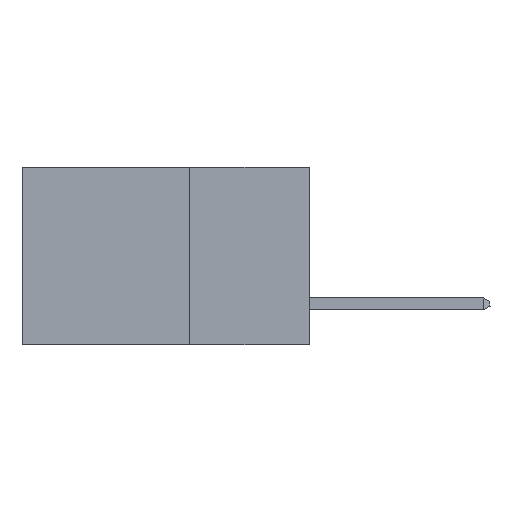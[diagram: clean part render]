
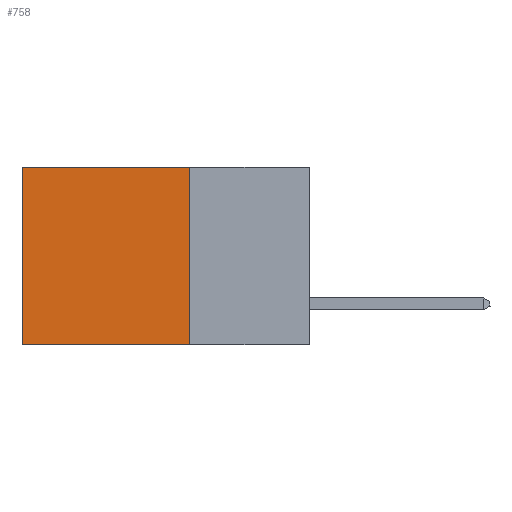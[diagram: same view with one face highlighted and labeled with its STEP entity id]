
A CAD part, left-side view. The second image highlights one B-rep face of the part: STEP entity #758.
In plain terms, the highlighted planar face has unit normal (-1, 0, 0).
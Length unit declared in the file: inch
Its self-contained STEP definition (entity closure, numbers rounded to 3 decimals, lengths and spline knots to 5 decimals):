
#326 = ORIENTED_EDGE ( 'NONE', *, *, #2407, .F. ) ;
#352 = VERTEX_POINT ( 'NONE', #2207 ) ;
#403 = CARTESIAN_POINT ( 'NONE',  ( 0.2875, 0.6, -0.37 ) ) ;
#758 = ADVANCED_FACE ( 'NONE', ( #17555 ), #6204, .F. ) ;
#1435 = VERTEX_POINT ( 'NONE', #6891 ) ;
#1757 = DIRECTION ( 'NONE',  ( 0., 0., -1. ) ) ;
#2174 = VECTOR ( 'NONE', #9789, 39.37008 ) ;
#2207 = CARTESIAN_POINT ( 'NONE',  ( 0.2875, 0.25, -0.37 ) ) ;
#2407 = EDGE_CURVE ( 'NONE', #352, #15777, #14944, .T. ) ;
#3303 = CARTESIAN_POINT ( 'NONE',  ( 0.2875, 0.25, 0. ) ) ;
#6085 = CARTESIAN_POINT ( 'NONE',  ( 0.2875, 0.25, 0. ) ) ;
#6204 = PLANE ( 'NONE',  #9492 ) ;
#6891 = CARTESIAN_POINT ( 'NONE',  ( 0.2875, 0.6, 0. ) ) ;
#6972 = LINE ( 'NONE', #3303, #2174 ) ;
#7022 = VECTOR ( 'NONE', #19555, 39.37008 ) ;
#7143 = DIRECTION ( 'NONE',  ( 0., 1., 0. ) ) ;
#7498 = EDGE_CURVE ( 'NONE', #1435, #15777, #16164, .T. ) ;
#8388 = CARTESIAN_POINT ( 'NONE',  ( 0.2875, 0.6, 0. ) ) ;
#9492 = AXIS2_PLACEMENT_3D ( 'NONE', #11681, #16072, #14426 ) ;
#9623 = CARTESIAN_POINT ( 'NONE',  ( 0.2875, 0.25, 0. ) ) ;
#9789 = DIRECTION ( 'NONE',  ( 0., 1., 0. ) ) ;
#10843 = EDGE_LOOP ( 'NONE', ( #18741, #326, #12575, #13223 ) ) ;
#11681 = CARTESIAN_POINT ( 'NONE',  ( 0.2875, 0.25, 0. ) ) ;
#12229 = VECTOR ( 'NONE', #1757, 39.37008 ) ;
#12575 = ORIENTED_EDGE ( 'NONE', *, *, #15576, .F. ) ;
#13223 = ORIENTED_EDGE ( 'NONE', *, *, #17467, .T. ) ;
#14426 = DIRECTION ( 'NONE',  ( 0., 0., -1. ) ) ;
#14427 = VERTEX_POINT ( 'NONE', #6085 ) ;
#14944 = LINE ( 'NONE', #16896, #15486 ) ;
#15486 = VECTOR ( 'NONE', #7143, 39.37008 ) ;
#15576 = EDGE_CURVE ( 'NONE', #14427, #352, #19356, .T. ) ;
#15777 = VERTEX_POINT ( 'NONE', #403 ) ;
#16072 = DIRECTION ( 'NONE',  ( 1., 0., 0. ) ) ;
#16164 = LINE ( 'NONE', #8388, #7022 ) ;
#16896 = CARTESIAN_POINT ( 'NONE',  ( 0.2875, 0.25, -0.37 ) ) ;
#17467 = EDGE_CURVE ( 'NONE', #14427, #1435, #6972, .T. ) ;
#17555 = FACE_OUTER_BOUND ( 'NONE', #10843, .T. ) ;
#18741 = ORIENTED_EDGE ( 'NONE', *, *, #7498, .T. ) ;
#19356 = LINE ( 'NONE', #9623, #12229 ) ;
#19555 = DIRECTION ( 'NONE',  ( 0., 0., -1. ) ) ;
